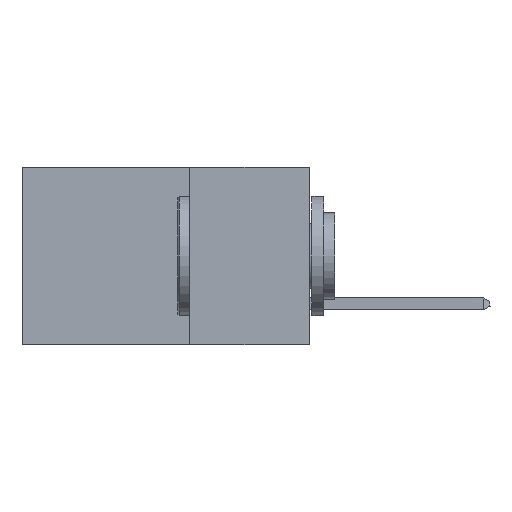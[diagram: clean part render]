
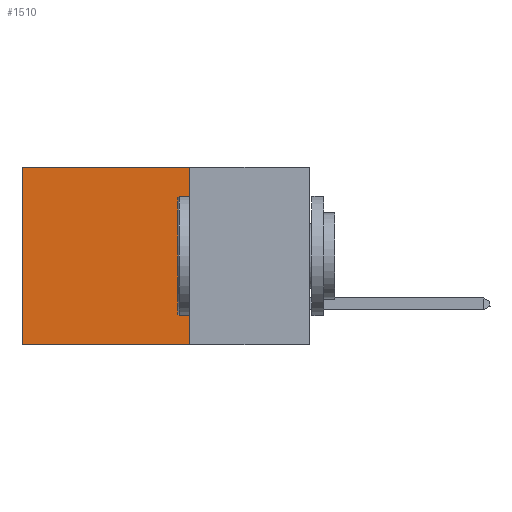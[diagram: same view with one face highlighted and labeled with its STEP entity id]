
A CAD part, left-side view. The second image highlights one B-rep face of the part: STEP entity #1510.
In plain terms, the highlighted planar face has unit normal (-1, 0, 0).
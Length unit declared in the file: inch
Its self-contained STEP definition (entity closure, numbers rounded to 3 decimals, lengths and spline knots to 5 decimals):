
#534 = DIRECTION ( 'NONE',  ( 0., 1., 0. ) ) ;
#592 = CARTESIAN_POINT ( 'NONE',  ( 0.2875, 0.6, 0. ) ) ;
#1088 = PLANE ( 'NONE',  #7517 ) ;
#1510 = ADVANCED_FACE ( 'NONE', ( #16391 ), #1088, .F. ) ;
#1716 = ORIENTED_EDGE ( 'NONE', *, *, #14119, .T. ) ;
#2330 = CARTESIAN_POINT ( 'NONE',  ( 0.2875, 0.25, -0.37 ) ) ;
#2736 = EDGE_CURVE ( 'NONE', #7670, #3288, #14586, .T. ) ;
#3288 = VERTEX_POINT ( 'NONE', #15194 ) ;
#3522 = CARTESIAN_POINT ( 'NONE',  ( 0.2875, 0.6, 0. ) ) ;
#3721 = DIRECTION ( 'NONE',  ( 0., 1., 0. ) ) ;
#3874 = DIRECTION ( 'NONE',  ( 0., 0., -1. ) ) ;
#4039 = VERTEX_POINT ( 'NONE', #9226 ) ;
#4793 = DIRECTION ( 'NONE',  ( 0., 0., -1. ) ) ;
#5837 = VECTOR ( 'NONE', #4793, 39.37008 ) ;
#7054 = ORIENTED_EDGE ( 'NONE', *, *, #12167, .F. ) ;
#7301 = EDGE_LOOP ( 'NONE', ( #17966, #7054, #11370, #1716 ) ) ;
#7517 = AXIS2_PLACEMENT_3D ( 'NONE', #15279, #12358, #12238 ) ;
#7670 = VERTEX_POINT ( 'NONE', #3522 ) ;
#7973 = CARTESIAN_POINT ( 'NONE',  ( 0.2875, 0.25, 0. ) ) ;
#8137 = VECTOR ( 'NONE', #3721, 39.37008 ) ;
#8947 = LINE ( 'NONE', #17248, #13927 ) ;
#9226 = CARTESIAN_POINT ( 'NONE',  ( 0.2875, 0.25, -0.37 ) ) ;
#9829 = VECTOR ( 'NONE', #3874, 39.37008 ) ;
#11370 = ORIENTED_EDGE ( 'NONE', *, *, #13590, .F. ) ;
#12133 = VERTEX_POINT ( 'NONE', #17566 ) ;
#12167 = EDGE_CURVE ( 'NONE', #4039, #3288, #17725, .T. ) ;
#12238 = DIRECTION ( 'NONE',  ( 0., 0., -1. ) ) ;
#12358 = DIRECTION ( 'NONE',  ( 1., 0., 0. ) ) ;
#13590 = EDGE_CURVE ( 'NONE', #12133, #4039, #15258, .T. ) ;
#13927 = VECTOR ( 'NONE', #534, 39.37008 ) ;
#14119 = EDGE_CURVE ( 'NONE', #12133, #7670, #8947, .T. ) ;
#14586 = LINE ( 'NONE', #592, #5837 ) ;
#15194 = CARTESIAN_POINT ( 'NONE',  ( 0.2875, 0.6, -0.37 ) ) ;
#15258 = LINE ( 'NONE', #7973, #9829 ) ;
#15279 = CARTESIAN_POINT ( 'NONE',  ( 0.2875, 0.25, 0. ) ) ;
#16391 = FACE_OUTER_BOUND ( 'NONE', #7301, .T. ) ;
#17248 = CARTESIAN_POINT ( 'NONE',  ( 0.2875, 0.25, 0. ) ) ;
#17566 = CARTESIAN_POINT ( 'NONE',  ( 0.2875, 0.25, 0. ) ) ;
#17725 = LINE ( 'NONE', #2330, #8137 ) ;
#17966 = ORIENTED_EDGE ( 'NONE', *, *, #2736, .T. ) ;
